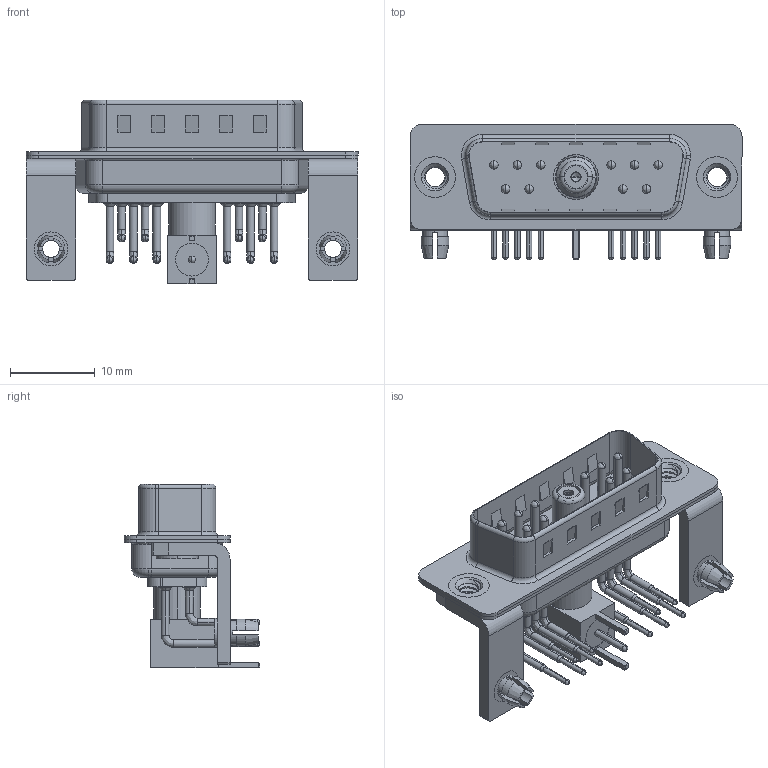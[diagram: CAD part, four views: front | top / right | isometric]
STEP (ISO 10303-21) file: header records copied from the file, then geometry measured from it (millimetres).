
FILE_DESCRIPTION (( 'STEP AP203' ), '1' );
FILE_NAME ('629-11W1240-7T3.STEP', '2022-05-06T21:58:08', ( '' ), ( '' ), 'SwSTEP 2.0', 'SolidWorks 2020', '' );
FILE_SCHEMA (( 'CONFIG_CONTROL_DESIGN' ));
Length unit declared in the file: millimetre
Products named in the file (17): Insulator RA Pin; 629Combo Stabilizer Bracket; 629Combo Shell Front_15 Contacts; Insulator Socket; 629Combo Contact Row 1; Co-Ax Jack Assy_RA; 629Combo Housing_11W1; Socket_RA; Co-Ax Jack_RA PC Tail; 629Combo Threaded Rivet_3; 629Combo Board Lock; Locking Collar; 629Combo Shell Rear_15 Contacts; RA Back Shell; 629Combo Contact Row 2; Insulator Socket 2; 629-11W1240-7T3
Assembly tree (27 placements, depth 3):
  629-11W1240-7T3
    629Combo Housing_11W1
    629Combo Shell Rear_15 Contacts
    629Combo Shell Front_15 Contacts
    629Combo Threaded Rivet_3  x2
    629Combo Stabilizer Bracket  x2
    629Combo Board Lock  x2
    Co-Ax Jack Assy_RA
      Co-Ax Jack_RA PC Tail
      Insulator Socket
      Insulator Socket 2
      Locking Collar
      Socket_RA
      RA Back Shell
      Insulator RA Pin
    629Combo Contact Row 1  x6
    629Combo Contact Row 2  x4
Bounding box: 39.2 x 16 x 21.71 mm (x, y, z)
Volume: 2515.3 mm3; surface area: 6875 mm2
Topology: 26 solids, 29 shells, 1737 faces, 4685 edges, 3027 vertices
Faces by surface type: plane 913, cylinder 614, cone 85, bspline 67, torus 56, sphere 2
Entity records: 28649 total; most frequent: CARTESIAN_POINT 6133, DIRECTION 4467, ORIENTED_EDGE 4126, EDGE_CURVE 2063, AXIS2_PLACEMENT_3D 1634, VERTEX_POINT 1328, LINE 1199, VECTOR 1199
